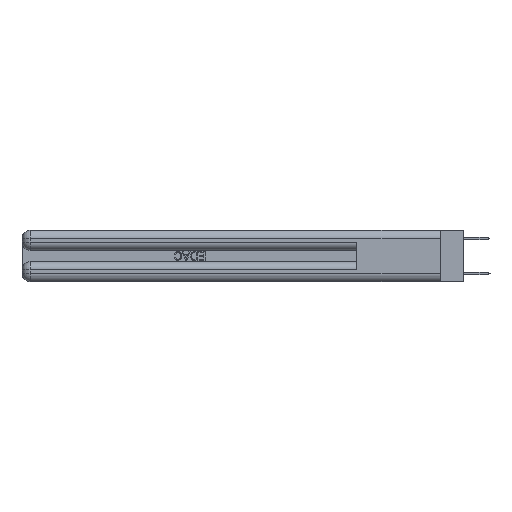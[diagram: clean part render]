
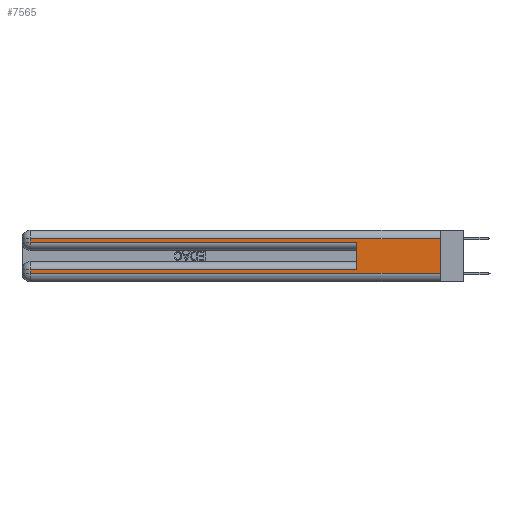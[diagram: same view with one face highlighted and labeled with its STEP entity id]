
A CAD part, left-side view. The second image highlights one B-rep face of the part: STEP entity #7565.
In plain terms, the highlighted planar face has unit normal (-1, 0, 0).
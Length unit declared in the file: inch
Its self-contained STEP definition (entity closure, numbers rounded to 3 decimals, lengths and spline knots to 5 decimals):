
#552 = DIRECTION ( 'NONE',  ( 0., 0., -1. ) ) ;
#1643 = VECTOR ( 'NONE', #28606, 39.37008 ) ;
#1891 = DIRECTION ( 'NONE',  ( 1., 0., 0. ) ) ;
#2485 = DIRECTION ( 'NONE',  ( 0., -1., 0. ) ) ;
#2689 = VERTEX_POINT ( 'NONE', #8722 ) ;
#2732 = EDGE_CURVE ( 'NONE', #24539, #21829, #19047, .T. ) ;
#2766 = CARTESIAN_POINT ( 'NONE',  ( 0., 0., 0.37 ) ) ;
#3183 = VECTOR ( 'NONE', #2485, 39.37008 ) ;
#3542 = ORIENTED_EDGE ( 'NONE', *, *, #13505, .F. ) ;
#3808 = EDGE_CURVE ( 'NONE', #21829, #14916, #27718, .T. ) ;
#4526 = VECTOR ( 'NONE', #22076, 39.37008 ) ;
#4839 = LINE ( 'NONE', #7497, #23406 ) ;
#6570 = ORIENTED_EDGE ( 'NONE', *, *, #15198, .T. ) ;
#6963 = ORIENTED_EDGE ( 'NONE', *, *, #31263, .T. ) ;
#7497 = CARTESIAN_POINT ( 'NONE',  ( 0., 2.94, 0.37 ) ) ;
#7565 = ADVANCED_FACE ( 'NONE', ( #19614 ), #30853, .F. ) ;
#7591 = CARTESIAN_POINT ( 'NONE',  ( 0., 2.94, 0.06 ) ) ;
#8038 = LINE ( 'NONE', #28049, #20165 ) ;
#8055 = ORIENTED_EDGE ( 'NONE', *, *, #22970, .T. ) ;
#8443 = VERTEX_POINT ( 'NONE', #27141 ) ;
#8722 = CARTESIAN_POINT ( 'NONE',  ( 0., 2.94, 0.085 ) ) ;
#9590 = ORIENTED_EDGE ( 'NONE', *, *, #3808, .T. ) ;
#10983 = LINE ( 'NONE', #17245, #4526 ) ;
#12980 = EDGE_CURVE ( 'NONE', #28137, #8443, #22512, .T. ) ;
#13505 = EDGE_CURVE ( 'NONE', #16341, #17605, #27404, .T. ) ;
#14008 = CARTESIAN_POINT ( 'NONE',  ( 0., 0.6, 0.145 ) ) ;
#14916 = VERTEX_POINT ( 'NONE', #17494 ) ;
#14929 = CARTESIAN_POINT ( 'NONE',  ( 0., 2.94, 0.31 ) ) ;
#14972 = AXIS2_PLACEMENT_3D ( 'NONE', #28462, #1891, #18867 ) ;
#15097 = CARTESIAN_POINT ( 'NONE',  ( 0., 2.94, 0.37 ) ) ;
#15198 = EDGE_CURVE ( 'NONE', #16341, #2689, #8038, .T. ) ;
#16341 = VERTEX_POINT ( 'NONE', #17120 ) ;
#17032 = CARTESIAN_POINT ( 'NONE',  ( 0., 0., 0.06 ) ) ;
#17120 = CARTESIAN_POINT ( 'NONE',  ( 0., 0.6, 0.085 ) ) ;
#17245 = CARTESIAN_POINT ( 'NONE',  ( 0., 0., 0.285 ) ) ;
#17328 = EDGE_CURVE ( 'NONE', #24539, #8443, #27595, .T. ) ;
#17494 = CARTESIAN_POINT ( 'NONE',  ( 0., 2.94, 0.285 ) ) ;
#17605 = VERTEX_POINT ( 'NONE', #20679 ) ;
#17951 = ORIENTED_EDGE ( 'NONE', *, *, #12980, .T. ) ;
#18290 = VECTOR ( 'NONE', #23319, 39.37008 ) ;
#18471 = CARTESIAN_POINT ( 'NONE',  ( 0., 0., 0.31 ) ) ;
#18867 = DIRECTION ( 'NONE',  ( 0., 0., -1. ) ) ;
#19047 = LINE ( 'NONE', #18471, #18290 ) ;
#19414 = ORIENTED_EDGE ( 'NONE', *, *, #17328, .F. ) ;
#19614 = FACE_OUTER_BOUND ( 'NONE', #30299, .T. ) ;
#20165 = VECTOR ( 'NONE', #23283, 39.37008 ) ;
#20679 = CARTESIAN_POINT ( 'NONE',  ( 0., 0.6, 0.285 ) ) ;
#21171 = VECTOR ( 'NONE', #29419, 39.37008 ) ;
#21829 = VERTEX_POINT ( 'NONE', #14929 ) ;
#22040 = VECTOR ( 'NONE', #552, 39.37008 ) ;
#22076 = DIRECTION ( 'NONE',  ( 0., -1., 0. ) ) ;
#22512 = LINE ( 'NONE', #17032, #3183 ) ;
#22970 = EDGE_CURVE ( 'NONE', #2689, #28137, #4839, .T. ) ;
#23283 = DIRECTION ( 'NONE',  ( 0., 1., 0. ) ) ;
#23319 = DIRECTION ( 'NONE',  ( 0., 1., 0. ) ) ;
#23406 = VECTOR ( 'NONE', #24525, 39.37008 ) ;
#24525 = DIRECTION ( 'NONE',  ( 0., 0., -1. ) ) ;
#24539 = VERTEX_POINT ( 'NONE', #28010 ) ;
#27141 = CARTESIAN_POINT ( 'NONE',  ( 0., 0., 0.06 ) ) ;
#27404 = LINE ( 'NONE', #14008, #1643 ) ;
#27595 = LINE ( 'NONE', #2766, #21171 ) ;
#27718 = LINE ( 'NONE', #15097, #22040 ) ;
#28010 = CARTESIAN_POINT ( 'NONE',  ( 0., 0., 0.31 ) ) ;
#28049 = CARTESIAN_POINT ( 'NONE',  ( 0., 0., 0.085 ) ) ;
#28137 = VERTEX_POINT ( 'NONE', #7591 ) ;
#28462 = CARTESIAN_POINT ( 'NONE',  ( 0., 0., 0.37 ) ) ;
#28606 = DIRECTION ( 'NONE',  ( 0., 0., 1. ) ) ;
#29419 = DIRECTION ( 'NONE',  ( 0., 0., -1. ) ) ;
#30299 = EDGE_LOOP ( 'NONE', ( #19414, #30719, #9590, #6963, #3542, #6570, #8055, #17951 ) ) ;
#30719 = ORIENTED_EDGE ( 'NONE', *, *, #2732, .T. ) ;
#30853 = PLANE ( 'NONE',  #14972 ) ;
#31263 = EDGE_CURVE ( 'NONE', #14916, #17605, #10983, .T. ) ;
